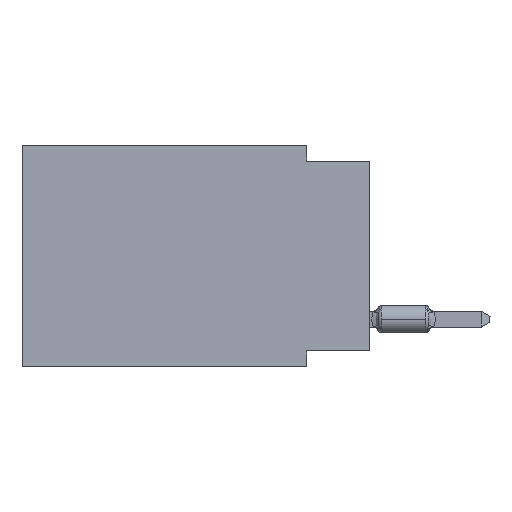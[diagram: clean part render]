
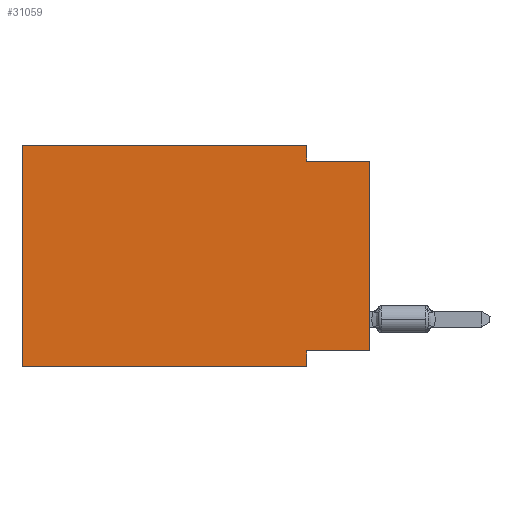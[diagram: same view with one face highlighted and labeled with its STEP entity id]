
A CAD part, left-side view. The second image highlights one B-rep face of the part: STEP entity #31059.
In plain terms, the highlighted planar face has unit normal (-1, 0, 0).
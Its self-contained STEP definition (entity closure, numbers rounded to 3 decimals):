
#505 = VERTEX_POINT ( 'NONE', #27426 ) ;
#929 = EDGE_CURVE ( 'NONE', #505, #11663, #13955, .T. ) ;
#979 = AXIS2_PLACEMENT_3D ( 'NONE', #25740, #12526, #15609 ) ;
#1652 = VERTEX_POINT ( 'NONE', #30597 ) ;
#2215 = VECTOR ( 'NONE', #3270, 1000. ) ;
#3223 = EDGE_LOOP ( 'NONE', ( #6425, #39401, #24248, #16987, #26562, #9916, #29384, #42517 ) ) ;
#3270 = DIRECTION ( 'NONE',  ( 0., 0., -1. ) ) ;
#3863 = EDGE_CURVE ( 'NONE', #21060, #37340, #9114, .T. ) ;
#4139 = CARTESIAN_POINT ( 'NONE',  ( 0., 2.54, -8.89 ) ) ;
#5047 = PLANE ( 'NONE',  #979 ) ;
#6425 = ORIENTED_EDGE ( 'NONE', *, *, #30806, .T. ) ;
#6579 = CARTESIAN_POINT ( 'NONE',  ( 0., 2.54, 0. ) ) ;
#6828 = DIRECTION ( 'NONE',  ( 0., -1., 0. ) ) ;
#6986 = EDGE_CURVE ( 'NONE', #1652, #505, #12339, .T. ) ;
#7961 = EDGE_CURVE ( 'NONE', #22256, #36503, #29496, .T. ) ;
#8155 = VERTEX_POINT ( 'NONE', #4139 ) ;
#9114 = LINE ( 'NONE', #37229, #19107 ) ;
#9916 = ORIENTED_EDGE ( 'NONE', *, *, #30085, .T. ) ;
#10129 = CARTESIAN_POINT ( 'NONE',  ( 0., 0., -8.255 ) ) ;
#11057 = VECTOR ( 'NONE', #16271, 1000. ) ;
#11663 = VERTEX_POINT ( 'NONE', #43031 ) ;
#12324 = FACE_OUTER_BOUND ( 'NONE', #3223, .T. ) ;
#12339 = LINE ( 'NONE', #18938, #11057 ) ;
#12526 = DIRECTION ( 'NONE',  ( 1., 0., 0. ) ) ;
#13951 = VECTOR ( 'NONE', #36563, 1000. ) ;
#13955 = LINE ( 'NONE', #41067, #25210 ) ;
#15609 = DIRECTION ( 'NONE',  ( 0., 0., -1. ) ) ;
#16271 = DIRECTION ( 'NONE',  ( 0., 0., 1. ) ) ;
#16987 = ORIENTED_EDGE ( 'NONE', *, *, #929, .F. ) ;
#17478 = DIRECTION ( 'NONE',  ( 0., -1., 0. ) ) ;
#17645 = EDGE_CURVE ( 'NONE', #11663, #21060, #36344, .T. ) ;
#18938 = CARTESIAN_POINT ( 'NONE',  ( 0., 13.97, 0. ) ) ;
#19093 = CARTESIAN_POINT ( 'NONE',  ( 0., 13.97, -8.89 ) ) ;
#19107 = VECTOR ( 'NONE', #6828, 1000. ) ;
#21060 = VERTEX_POINT ( 'NONE', #42217 ) ;
#22256 = VERTEX_POINT ( 'NONE', #38926 ) ;
#22306 = LINE ( 'NONE', #41725, #28883 ) ;
#22377 = LINE ( 'NONE', #19093, #34004 ) ;
#24248 = ORIENTED_EDGE ( 'NONE', *, *, #17645, .F. ) ;
#24963 = CARTESIAN_POINT ( 'NONE',  ( 0., 0., -0.635 ) ) ;
#25210 = VECTOR ( 'NONE', #17478, 1000. ) ;
#25740 = CARTESIAN_POINT ( 'NONE',  ( 0., 13.97, 0. ) ) ;
#26442 = LINE ( 'NONE', #33934, #40355 ) ;
#26465 = EDGE_CURVE ( 'NONE', #36503, #8155, #22306, .T. ) ;
#26562 = ORIENTED_EDGE ( 'NONE', *, *, #6986, .F. ) ;
#27426 = CARTESIAN_POINT ( 'NONE',  ( 0., 13.97, 0. ) ) ;
#28883 = VECTOR ( 'NONE', #34881, 1000. ) ;
#29384 = ORIENTED_EDGE ( 'NONE', *, *, #26465, .F. ) ;
#29496 = LINE ( 'NONE', #10129, #13951 ) ;
#30085 = EDGE_CURVE ( 'NONE', #1652, #8155, #22377, .T. ) ;
#30597 = CARTESIAN_POINT ( 'NONE',  ( 0., 13.97, -8.89 ) ) ;
#30806 = EDGE_CURVE ( 'NONE', #22256, #37340, #26442, .T. ) ;
#31059 = ADVANCED_FACE ( 'NONE', ( #12324 ), #5047, .F. ) ;
#31680 = CARTESIAN_POINT ( 'NONE',  ( 0., 2.54, -8.255 ) ) ;
#33934 = CARTESIAN_POINT ( 'NONE',  ( 0., 0., 0. ) ) ;
#34004 = VECTOR ( 'NONE', #35830, 1000. ) ;
#34881 = DIRECTION ( 'NONE',  ( 0., 0., -1. ) ) ;
#35830 = DIRECTION ( 'NONE',  ( 0., -1., 0. ) ) ;
#36344 = LINE ( 'NONE', #6579, #2215 ) ;
#36503 = VERTEX_POINT ( 'NONE', #31680 ) ;
#36563 = DIRECTION ( 'NONE',  ( 0., 1., 0. ) ) ;
#37229 = CARTESIAN_POINT ( 'NONE',  ( 0., 0., -0.635 ) ) ;
#37340 = VERTEX_POINT ( 'NONE', #24963 ) ;
#38926 = CARTESIAN_POINT ( 'NONE',  ( 0., 0., -8.255 ) ) ;
#39401 = ORIENTED_EDGE ( 'NONE', *, *, #3863, .F. ) ;
#39889 = DIRECTION ( 'NONE',  ( 0., 0., 1. ) ) ;
#40355 = VECTOR ( 'NONE', #39889, 1000. ) ;
#41067 = CARTESIAN_POINT ( 'NONE',  ( 0., 13.97, 0. ) ) ;
#41725 = CARTESIAN_POINT ( 'NONE',  ( 0., 2.54, -8.89 ) ) ;
#42217 = CARTESIAN_POINT ( 'NONE',  ( 0., 2.54, -0.635 ) ) ;
#42517 = ORIENTED_EDGE ( 'NONE', *, *, #7961, .F. ) ;
#43031 = CARTESIAN_POINT ( 'NONE',  ( 0., 2.54, 0. ) ) ;
